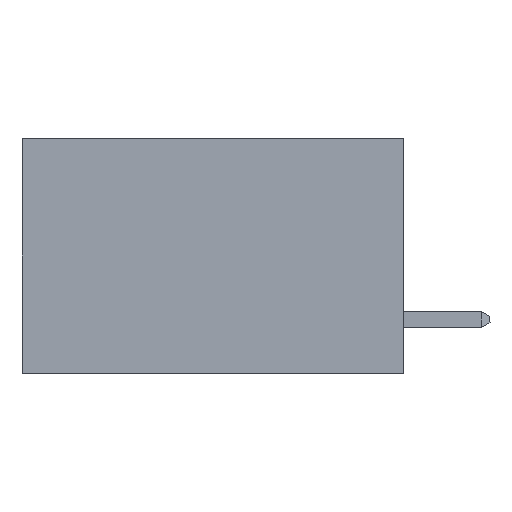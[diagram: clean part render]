
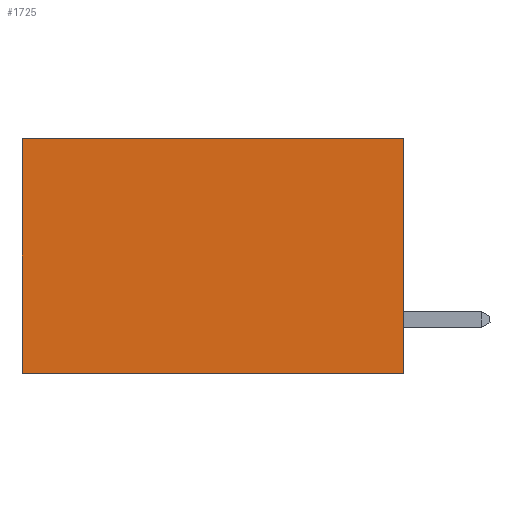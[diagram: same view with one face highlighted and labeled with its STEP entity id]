
A CAD part, left-side view. The second image highlights one B-rep face of the part: STEP entity #1725.
In plain terms, the highlighted planar face has unit normal (-1, 0, 0).
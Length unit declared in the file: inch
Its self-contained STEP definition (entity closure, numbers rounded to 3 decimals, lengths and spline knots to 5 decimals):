
#75 = ORIENTED_EDGE ( 'NONE', *, *, #9704, .T. ) ;
#578 = VERTEX_POINT ( 'NONE', #5336 ) ;
#1287 = EDGE_CURVE ( 'NONE', #9245, #578, #2670, .T. ) ;
#1725 = ADVANCED_FACE ( 'NONE', ( #7094 ), #3169, .F. ) ;
#1838 = VECTOR ( 'NONE', #5289, 39.37008 ) ;
#2107 = LINE ( 'NONE', #9876, #8214 ) ;
#2523 = CARTESIAN_POINT ( 'NONE',  ( 0.2875, 0., -0.37 ) ) ;
#2670 = LINE ( 'NONE', #5503, #8691 ) ;
#2761 = CARTESIAN_POINT ( 'NONE',  ( 0.2875, 0., 0. ) ) ;
#3169 = PLANE ( 'NONE',  #5679 ) ;
#3765 = CARTESIAN_POINT ( 'NONE',  ( 0.2875, 0., 0. ) ) ;
#4312 = LINE ( 'NONE', #2761, #1838 ) ;
#4711 = EDGE_CURVE ( 'NONE', #7294, #9245, #4312, .T. ) ;
#5027 = ORIENTED_EDGE ( 'NONE', *, *, #4711, .F. ) ;
#5081 = DIRECTION ( 'NONE',  ( 0., 0., -1. ) ) ;
#5084 = ORIENTED_EDGE ( 'NONE', *, *, #1287, .F. ) ;
#5289 = DIRECTION ( 'NONE',  ( 0., 0., -1. ) ) ;
#5293 = CARTESIAN_POINT ( 'NONE',  ( 0.2875, 0., 0. ) ) ;
#5307 = DIRECTION ( 'NONE',  ( 1., 0., 0. ) ) ;
#5336 = CARTESIAN_POINT ( 'NONE',  ( 0.2875, 0.6, -0.37 ) ) ;
#5440 = DIRECTION ( 'NONE',  ( 0., 0., -1. ) ) ;
#5501 = ORIENTED_EDGE ( 'NONE', *, *, #8219, .T. ) ;
#5503 = CARTESIAN_POINT ( 'NONE',  ( 0.2875, 0., -0.37 ) ) ;
#5528 = CARTESIAN_POINT ( 'NONE',  ( 0.2875, 0., 0. ) ) ;
#5679 = AXIS2_PLACEMENT_3D ( 'NONE', #5293, #5307, #5081 ) ;
#6537 = CARTESIAN_POINT ( 'NONE',  ( 0.2875, 0.6, 0. ) ) ;
#6964 = DIRECTION ( 'NONE',  ( 0., 1., 0. ) ) ;
#7007 = DIRECTION ( 'NONE',  ( 0., 1., 0. ) ) ;
#7094 = FACE_OUTER_BOUND ( 'NONE', #9819, .T. ) ;
#7294 = VERTEX_POINT ( 'NONE', #5528 ) ;
#7442 = LINE ( 'NONE', #3765, #10131 ) ;
#7651 = VERTEX_POINT ( 'NONE', #6537 ) ;
#8214 = VECTOR ( 'NONE', #5440, 39.37008 ) ;
#8219 = EDGE_CURVE ( 'NONE', #7294, #7651, #7442, .T. ) ;
#8691 = VECTOR ( 'NONE', #6964, 39.37008 ) ;
#9245 = VERTEX_POINT ( 'NONE', #2523 ) ;
#9704 = EDGE_CURVE ( 'NONE', #7651, #578, #2107, .T. ) ;
#9819 = EDGE_LOOP ( 'NONE', ( #75, #5084, #5027, #5501 ) ) ;
#9876 = CARTESIAN_POINT ( 'NONE',  ( 0.2875, 0.6, 0. ) ) ;
#10131 = VECTOR ( 'NONE', #7007, 39.37008 ) ;
